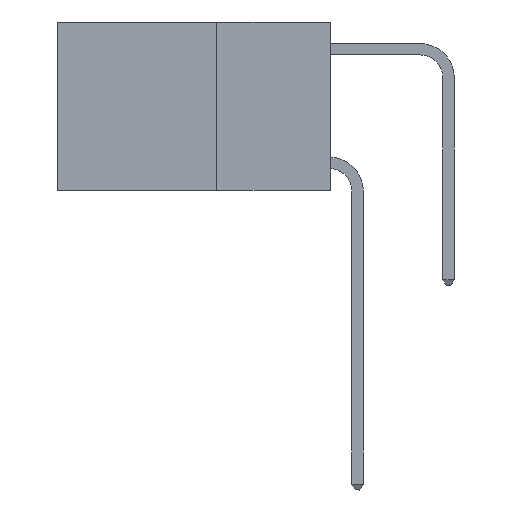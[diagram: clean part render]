
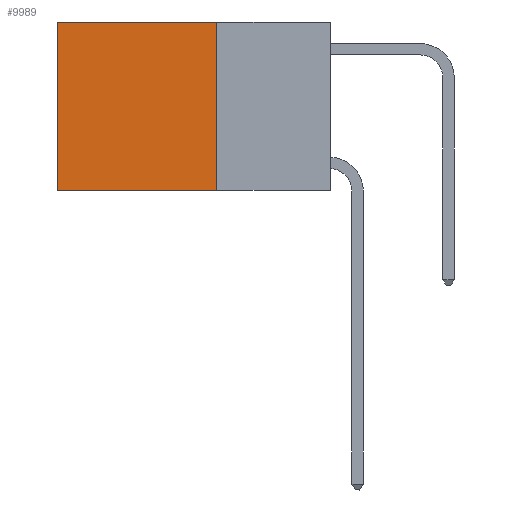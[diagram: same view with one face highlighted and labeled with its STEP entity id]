
A CAD part, left-side view. The second image highlights one B-rep face of the part: STEP entity #9989.
In plain terms, the highlighted planar face has unit normal (-1, 0, 0).
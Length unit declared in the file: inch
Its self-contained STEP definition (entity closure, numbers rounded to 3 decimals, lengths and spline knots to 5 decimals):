
#118 = DIRECTION ( 'NONE',  ( 0., 1., 0. ) ) ;
#500 = VERTEX_POINT ( 'NONE', #3692 ) ;
#796 = DIRECTION ( 'NONE',  ( 1., 0., 0. ) ) ;
#817 = EDGE_CURVE ( 'NONE', #1193, #8465, #2394, .T. ) ;
#1111 = EDGE_CURVE ( 'NONE', #3489, #8465, #11603, .T. ) ;
#1193 = VERTEX_POINT ( 'NONE', #11934 ) ;
#1974 = CARTESIAN_POINT ( 'NONE',  ( 0.2625, 0.25, 0. ) ) ;
#2394 = LINE ( 'NONE', #7502, #9263 ) ;
#2933 = LINE ( 'NONE', #1974, #11710 ) ;
#3202 = FACE_OUTER_BOUND ( 'NONE', #7507, .T. ) ;
#3489 = VERTEX_POINT ( 'NONE', #3691 ) ;
#3691 = CARTESIAN_POINT ( 'NONE',  ( 0.2625, 0.6, 0. ) ) ;
#3692 = CARTESIAN_POINT ( 'NONE',  ( 0.2625, 0.25, 0. ) ) ;
#3779 = ORIENTED_EDGE ( 'NONE', *, *, #9285, .T. ) ;
#4407 = ORIENTED_EDGE ( 'NONE', *, *, #1111, .T. ) ;
#4643 = EDGE_CURVE ( 'NONE', #500, #1193, #2933, .T. ) ;
#5085 = CARTESIAN_POINT ( 'NONE',  ( 0.2625, 0.6, 0. ) ) ;
#6145 = DIRECTION ( 'NONE',  ( 0., 0., -1. ) ) ;
#6625 = CARTESIAN_POINT ( 'NONE',  ( 0.2625, 0.25, 0. ) ) ;
#6639 = ORIENTED_EDGE ( 'NONE', *, *, #4643, .F. ) ;
#7502 = CARTESIAN_POINT ( 'NONE',  ( 0.2625, 0.25, -0.37 ) ) ;
#7507 = EDGE_LOOP ( 'NONE', ( #4407, #8417, #6639, #3779 ) ) ;
#8259 = DIRECTION ( 'NONE',  ( 0., 0., -1. ) ) ;
#8313 = DIRECTION ( 'NONE',  ( 0., 1., 0. ) ) ;
#8417 = ORIENTED_EDGE ( 'NONE', *, *, #817, .F. ) ;
#8442 = PLANE ( 'NONE',  #10022 ) ;
#8465 = VERTEX_POINT ( 'NONE', #8719 ) ;
#8719 = CARTESIAN_POINT ( 'NONE',  ( 0.2625, 0.6, -0.37 ) ) ;
#8791 = VECTOR ( 'NONE', #118, 39.37008 ) ;
#9263 = VECTOR ( 'NONE', #8313, 39.37008 ) ;
#9285 = EDGE_CURVE ( 'NONE', #500, #3489, #11591, .T. ) ;
#9593 = DIRECTION ( 'NONE',  ( 0., 0., -1. ) ) ;
#9989 = ADVANCED_FACE ( 'NONE', ( #3202 ), #8442, .F. ) ;
#10022 = AXIS2_PLACEMENT_3D ( 'NONE', #6625, #796, #9593 ) ;
#11029 = VECTOR ( 'NONE', #6145, 39.37008 ) ;
#11591 = LINE ( 'NONE', #11698, #8791 ) ;
#11603 = LINE ( 'NONE', #5085, #11029 ) ;
#11698 = CARTESIAN_POINT ( 'NONE',  ( 0.2625, 0.25, 0. ) ) ;
#11710 = VECTOR ( 'NONE', #8259, 39.37008 ) ;
#11934 = CARTESIAN_POINT ( 'NONE',  ( 0.2625, 0.25, -0.37 ) ) ;
